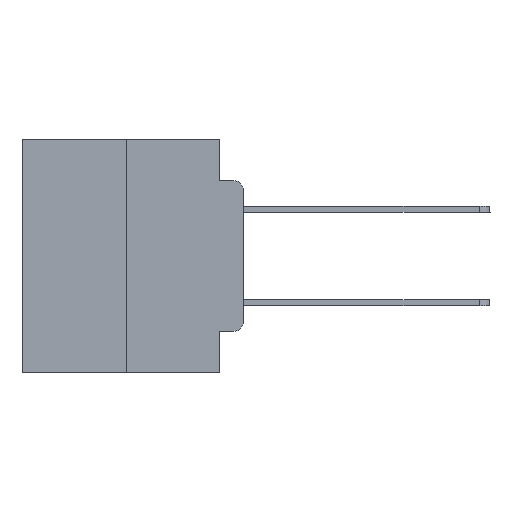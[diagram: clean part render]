
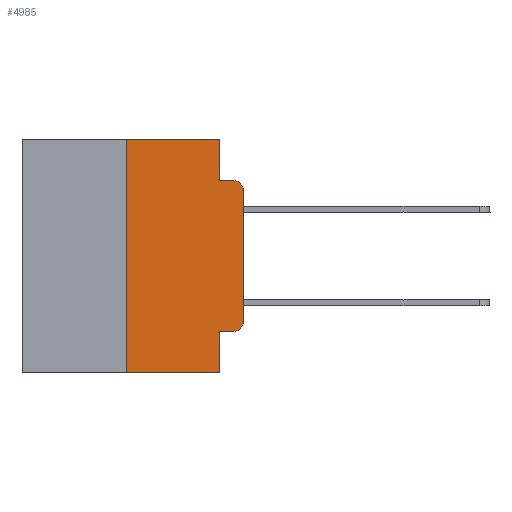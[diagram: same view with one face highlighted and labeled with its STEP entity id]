
A CAD part, left-side view. The second image highlights one B-rep face of the part: STEP entity #4985.
In plain terms, the highlighted planar face has unit normal (-1, 0, 0).
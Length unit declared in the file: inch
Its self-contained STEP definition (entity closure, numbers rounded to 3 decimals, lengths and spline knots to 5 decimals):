
#779 = DIRECTION ( 'NONE',  ( 0., -1., 0. ) ) ;
#2223 = DIRECTION ( 'NONE',  ( 0., 0., -1. ) ) ;
#2233 = VECTOR ( 'NONE', #23154, 39.37008 ) ;
#2468 = EDGE_CURVE ( 'NONE', #10132, #21990, #15490, .T. ) ;
#2790 = DIRECTION ( 'NONE',  ( 0., 0., -1. ) ) ;
#3275 = ORIENTED_EDGE ( 'NONE', *, *, #5621, .T. ) ;
#3363 = VERTEX_POINT ( 'NONE', #5478 ) ;
#3868 = EDGE_CURVE ( 'NONE', #7721, #5063, #15424, .T. ) ;
#4452 = VERTEX_POINT ( 'NONE', #6020 ) ;
#4590 = DIRECTION ( 'NONE',  ( 0., 0., 1. ) ) ;
#4671 = CARTESIAN_POINT ( 'NONE',  ( 0., 0.051, 0. ) ) ;
#4864 = VERTEX_POINT ( 'NONE', #13373 ) ;
#4940 = CARTESIAN_POINT ( 'NONE',  ( 0., 0.051, 0. ) ) ;
#4985 = ADVANCED_FACE ( 'NONE', ( #12475 ), #15510, .F. ) ;
#5060 = CARTESIAN_POINT ( 'NONE',  ( 0., 0.051, -0.0885 ) ) ;
#5063 = VERTEX_POINT ( 'NONE', #17210 ) ;
#5391 = ORIENTED_EDGE ( 'NONE', *, *, #6220, .F. ) ;
#5400 = EDGE_CURVE ( 'NONE', #10132, #5683, #25286, .T. ) ;
#5431 = EDGE_CURVE ( 'NONE', #5063, #3363, #18239, .T. ) ;
#5478 = CARTESIAN_POINT ( 'NONE',  ( 0., 0., -0.3915 ) ) ;
#5598 = CARTESIAN_POINT ( 'NONE',  ( 0., 0.473, 0. ) ) ;
#5621 = EDGE_CURVE ( 'NONE', #3363, #17333, #11152, .T. ) ;
#5683 = VERTEX_POINT ( 'NONE', #17980 ) ;
#6020 = CARTESIAN_POINT ( 'NONE',  ( 0., 0.051, -0.0885 ) ) ;
#6037 = AXIS2_PLACEMENT_3D ( 'NONE', #16397, #6355, #2223 ) ;
#6220 = EDGE_CURVE ( 'NONE', #4864, #4452, #18500, .T. ) ;
#6355 = DIRECTION ( 'NONE',  ( -1., 0., 0. ) ) ;
#6569 = CARTESIAN_POINT ( 'NONE',  ( 0., 0.02, -0.3915 ) ) ;
#6591 = VECTOR ( 'NONE', #9395, 39.37008 ) ;
#6604 = CARTESIAN_POINT ( 'NONE',  ( 0., 0., -0.1085 ) ) ;
#7721 = VERTEX_POINT ( 'NONE', #21957 ) ;
#7973 = VECTOR ( 'NONE', #4590, 39.37008 ) ;
#8237 = ORIENTED_EDGE ( 'NONE', *, *, #5431, .T. ) ;
#8676 = CARTESIAN_POINT ( 'NONE',  ( 0., 0.051, -0.4115 ) ) ;
#8827 = EDGE_CURVE ( 'NONE', #7721, #21990, #20870, .T. ) ;
#8944 = DIRECTION ( 'NONE',  ( 0., -1., 0. ) ) ;
#9395 = DIRECTION ( 'NONE',  ( 0., -1., 0. ) ) ;
#9444 = LINE ( 'NONE', #5060, #25801 ) ;
#10132 = VERTEX_POINT ( 'NONE', #12708 ) ;
#10144 = VERTEX_POINT ( 'NONE', #22914 ) ;
#10529 = CARTESIAN_POINT ( 'NONE',  ( 0., 0.25, 0. ) ) ;
#11152 = LINE ( 'NONE', #19410, #21739 ) ;
#12050 = LINE ( 'NONE', #5598, #6591 ) ;
#12079 = ORIENTED_EDGE ( 'NONE', *, *, #15220, .F. ) ;
#12475 = FACE_OUTER_BOUND ( 'NONE', #22254, .T. ) ;
#12708 = CARTESIAN_POINT ( 'NONE',  ( 0., 0.25, -0.5 ) ) ;
#13373 = CARTESIAN_POINT ( 'NONE',  ( 0., 0.051, 0. ) ) ;
#13709 = AXIS2_PLACEMENT_3D ( 'NONE', #6569, #14916, #16619 ) ;
#14916 = DIRECTION ( 'NONE',  ( -1., 0., 0. ) ) ;
#14917 = ORIENTED_EDGE ( 'NONE', *, *, #8827, .F. ) ;
#14967 = ORIENTED_EDGE ( 'NONE', *, *, #5400, .F. ) ;
#15220 = EDGE_CURVE ( 'NONE', #5683, #4864, #12050, .T. ) ;
#15311 = ORIENTED_EDGE ( 'NONE', *, *, #22573, .F. ) ;
#15348 = CARTESIAN_POINT ( 'NONE',  ( 0., 0.473, -0.5 ) ) ;
#15424 = LINE ( 'NONE', #8676, #21838 ) ;
#15490 = LINE ( 'NONE', #15348, #20957 ) ;
#15510 = PLANE ( 'NONE',  #20750 ) ;
#15664 = CARTESIAN_POINT ( 'NONE',  ( 0., 0.051, -0.5 ) ) ;
#16397 = CARTESIAN_POINT ( 'NONE',  ( 0., 0.02, -0.1085 ) ) ;
#16619 = DIRECTION ( 'NONE',  ( 0., 0., -1. ) ) ;
#17210 = CARTESIAN_POINT ( 'NONE',  ( 0., 0.02, -0.4115 ) ) ;
#17333 = VERTEX_POINT ( 'NONE', #6604 ) ;
#17980 = CARTESIAN_POINT ( 'NONE',  ( 0., 0.25, 0. ) ) ;
#18239 = CIRCLE ( 'NONE', #13709, 0.02 ) ;
#18283 = ORIENTED_EDGE ( 'NONE', *, *, #19799, .T. ) ;
#18500 = LINE ( 'NONE', #4671, #20429 ) ;
#18620 = CIRCLE ( 'NONE', #6037, 0.02 ) ;
#19410 = CARTESIAN_POINT ( 'NONE',  ( 0., 0., 0. ) ) ;
#19799 = EDGE_CURVE ( 'NONE', #17333, #10144, #18620, .T. ) ;
#20429 = VECTOR ( 'NONE', #2790, 39.37008 ) ;
#20750 = AXIS2_PLACEMENT_3D ( 'NONE', #25815, #25360, #25011 ) ;
#20870 = LINE ( 'NONE', #4940, #2233 ) ;
#20957 = VECTOR ( 'NONE', #779, 39.37008 ) ;
#21739 = VECTOR ( 'NONE', #23257, 39.37008 ) ;
#21838 = VECTOR ( 'NONE', #23270, 39.37008 ) ;
#21957 = CARTESIAN_POINT ( 'NONE',  ( 0., 0.051, -0.4115 ) ) ;
#21990 = VERTEX_POINT ( 'NONE', #15664 ) ;
#22254 = EDGE_LOOP ( 'NONE', ( #3275, #18283, #15311, #5391, #12079, #14967, #23574, #14917, #25291, #8237 ) ) ;
#22573 = EDGE_CURVE ( 'NONE', #4452, #10144, #9444, .T. ) ;
#22914 = CARTESIAN_POINT ( 'NONE',  ( 0., 0.02, -0.0885 ) ) ;
#23154 = DIRECTION ( 'NONE',  ( 0., 0., -1. ) ) ;
#23257 = DIRECTION ( 'NONE',  ( 0., 0., 1. ) ) ;
#23270 = DIRECTION ( 'NONE',  ( 0., -1., 0. ) ) ;
#23574 = ORIENTED_EDGE ( 'NONE', *, *, #2468, .T. ) ;
#25011 = DIRECTION ( 'NONE',  ( 0., 0., -1. ) ) ;
#25286 = LINE ( 'NONE', #10529, #7973 ) ;
#25291 = ORIENTED_EDGE ( 'NONE', *, *, #3868, .T. ) ;
#25360 = DIRECTION ( 'NONE',  ( 1., 0., 0. ) ) ;
#25801 = VECTOR ( 'NONE', #8944, 39.37008 ) ;
#25815 = CARTESIAN_POINT ( 'NONE',  ( 0., 0.473, 0. ) ) ;
